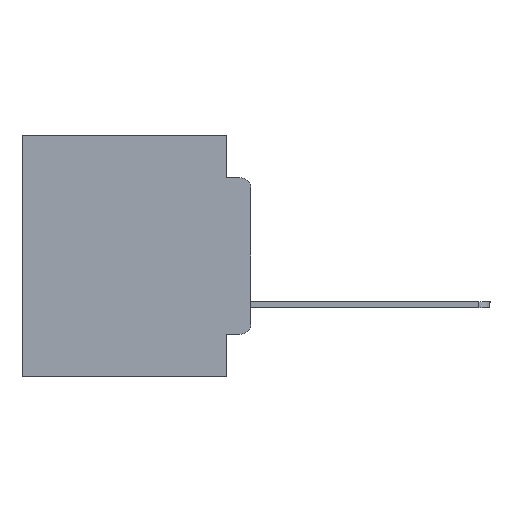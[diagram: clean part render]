
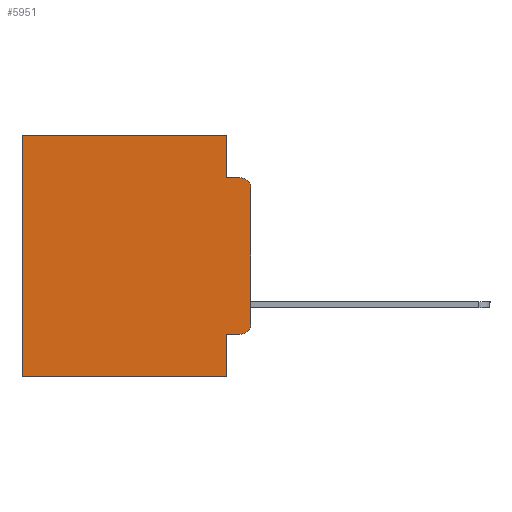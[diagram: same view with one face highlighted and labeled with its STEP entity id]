
A CAD part, left-side view. The second image highlights one B-rep face of the part: STEP entity #5951.
In plain terms, the highlighted planar face has unit normal (-1, 0, 0).
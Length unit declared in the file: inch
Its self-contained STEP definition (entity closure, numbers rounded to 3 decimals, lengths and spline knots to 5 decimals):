
#477 = CARTESIAN_POINT ( 'NONE',  ( 0.298, 0.051, -0.5 ) ) ;
#1164 = VECTOR ( 'NONE', #3734, 39.37008 ) ;
#1680 = ORIENTED_EDGE ( 'NONE', *, *, #22626, .F. ) ;
#1765 = VECTOR ( 'NONE', #3076, 39.37008 ) ;
#2395 = CARTESIAN_POINT ( 'NONE',  ( 0.298, 0.473, -0.5 ) ) ;
#2479 = DIRECTION ( 'NONE',  ( 0., 0., -1. ) ) ;
#2806 = VERTEX_POINT ( 'NONE', #5251 ) ;
#3076 = DIRECTION ( 'NONE',  ( 0., -1., 0. ) ) ;
#3149 = EDGE_CURVE ( 'NONE', #2806, #12710, #28818, .T. ) ;
#3280 = DIRECTION ( 'NONE',  ( -1., 0., 0. ) ) ;
#3322 = CARTESIAN_POINT ( 'NONE',  ( 0.298, 0.051, 0. ) ) ;
#3734 = DIRECTION ( 'NONE',  ( 0., 0., -1. ) ) ;
#3807 = PLANE ( 'NONE',  #22149 ) ;
#4066 = ORIENTED_EDGE ( 'NONE', *, *, #28423, .F. ) ;
#4563 = CARTESIAN_POINT ( 'NONE',  ( 0.298, 0., -0.3915 ) ) ;
#4841 = EDGE_CURVE ( 'NONE', #13880, #23480, #18587, .T. ) ;
#5045 = DIRECTION ( 'NONE',  ( -1., 0., 0. ) ) ;
#5251 = CARTESIAN_POINT ( 'NONE',  ( 0.298, 0., -0.1085 ) ) ;
#5495 = CARTESIAN_POINT ( 'NONE',  ( 0.298, 0., -0.5 ) ) ;
#5843 = DIRECTION ( 'NONE',  ( 0., 0., -1. ) ) ;
#5951 = ADVANCED_FACE ( 'NONE', ( #17304 ), #3807, .F. ) ;
#6473 = EDGE_CURVE ( 'NONE', #12694, #21999, #13450, .T. ) ;
#7042 = LINE ( 'NONE', #15993, #1765 ) ;
#9878 = AXIS2_PLACEMENT_3D ( 'NONE', #14836, #3280, #23289 ) ;
#10331 = CIRCLE ( 'NONE', #9878, 0.02 ) ;
#10466 = CARTESIAN_POINT ( 'NONE',  ( 0.298, 0.02, -0.0885 ) ) ;
#10479 = EDGE_CURVE ( 'NONE', #2806, #23607, #28975, .T. ) ;
#10748 = CARTESIAN_POINT ( 'NONE',  ( 0.298, 0., 0. ) ) ;
#11320 = EDGE_CURVE ( 'NONE', #13880, #13635, #14856, .T. ) ;
#12081 = ORIENTED_EDGE ( 'NONE', *, *, #4841, .T. ) ;
#12694 = VERTEX_POINT ( 'NONE', #14717 ) ;
#12710 = VERTEX_POINT ( 'NONE', #10466 ) ;
#12803 = LINE ( 'NONE', #10748, #27935 ) ;
#13104 = ORIENTED_EDGE ( 'NONE', *, *, #25873, .T. ) ;
#13133 = VECTOR ( 'NONE', #16226, 39.37008 ) ;
#13152 = CARTESIAN_POINT ( 'NONE',  ( 0.298, 0.473, 0. ) ) ;
#13450 = LINE ( 'NONE', #13152, #14121 ) ;
#13472 = CARTESIAN_POINT ( 'NONE',  ( 0.298, 0., 0. ) ) ;
#13635 = VERTEX_POINT ( 'NONE', #477 ) ;
#13880 = VERTEX_POINT ( 'NONE', #21483 ) ;
#14121 = VECTOR ( 'NONE', #22615, 39.37008 ) ;
#14569 = EDGE_CURVE ( 'NONE', #13635, #21999, #23181, .T. ) ;
#14702 = DIRECTION ( 'NONE',  ( 0., 1., 0. ) ) ;
#14717 = CARTESIAN_POINT ( 'NONE',  ( 0.298, 0.473, 0. ) ) ;
#14836 = CARTESIAN_POINT ( 'NONE',  ( 0.298, 0.02, -0.3915 ) ) ;
#14856 = LINE ( 'NONE', #17381, #1164 ) ;
#15084 = CARTESIAN_POINT ( 'NONE',  ( 0.298, 0., 0. ) ) ;
#15254 = CARTESIAN_POINT ( 'NONE',  ( 0.298, 0.02, -0.4115 ) ) ;
#15299 = ORIENTED_EDGE ( 'NONE', *, *, #14569, .F. ) ;
#15993 = CARTESIAN_POINT ( 'NONE',  ( 0.298, 0.051, -0.0885 ) ) ;
#16226 = DIRECTION ( 'NONE',  ( 0., -1., 0. ) ) ;
#16483 = DIRECTION ( 'NONE',  ( 0., 0., -1. ) ) ;
#17098 = ORIENTED_EDGE ( 'NONE', *, *, #6473, .T. ) ;
#17168 = CARTESIAN_POINT ( 'NONE',  ( 0.298, 0.051, -0.0885 ) ) ;
#17304 = FACE_OUTER_BOUND ( 'NONE', #22962, .T. ) ;
#17381 = CARTESIAN_POINT ( 'NONE',  ( 0.298, 0.051, 0. ) ) ;
#18193 = EDGE_CURVE ( 'NONE', #22625, #12694, #12803, .T. ) ;
#18293 = VECTOR ( 'NONE', #18473, 39.37008 ) ;
#18456 = AXIS2_PLACEMENT_3D ( 'NONE', #27041, #5045, #16483 ) ;
#18473 = DIRECTION ( 'NONE',  ( 0., 0., -1. ) ) ;
#18587 = LINE ( 'NONE', #25391, #13133 ) ;
#18737 = DIRECTION ( 'NONE',  ( 0., 1., 0. ) ) ;
#20976 = LINE ( 'NONE', #3322, #18293 ) ;
#21149 = CARTESIAN_POINT ( 'NONE',  ( 0.298, 0.051, 0. ) ) ;
#21483 = CARTESIAN_POINT ( 'NONE',  ( 0.298, 0.051, -0.4115 ) ) ;
#21999 = VERTEX_POINT ( 'NONE', #2395 ) ;
#22149 = AXIS2_PLACEMENT_3D ( 'NONE', #15084, #24113, #5843 ) ;
#22615 = DIRECTION ( 'NONE',  ( 0., 0., -1. ) ) ;
#22625 = VERTEX_POINT ( 'NONE', #21149 ) ;
#22626 = EDGE_CURVE ( 'NONE', #25217, #12710, #7042, .T. ) ;
#22962 = EDGE_LOOP ( 'NONE', ( #27747, #25265, #1680, #4066, #23292, #17098, #15299, #26859, #12081, #13104 ) ) ;
#23181 = LINE ( 'NONE', #5495, #26174 ) ;
#23289 = DIRECTION ( 'NONE',  ( 0., 0., -1. ) ) ;
#23292 = ORIENTED_EDGE ( 'NONE', *, *, #18193, .T. ) ;
#23480 = VERTEX_POINT ( 'NONE', #15254 ) ;
#23607 = VERTEX_POINT ( 'NONE', #4563 ) ;
#24113 = DIRECTION ( 'NONE',  ( 1., 0., 0. ) ) ;
#25217 = VERTEX_POINT ( 'NONE', #17168 ) ;
#25265 = ORIENTED_EDGE ( 'NONE', *, *, #3149, .T. ) ;
#25391 = CARTESIAN_POINT ( 'NONE',  ( 0.298, 0.051, -0.4115 ) ) ;
#25873 = EDGE_CURVE ( 'NONE', #23480, #23607, #10331, .T. ) ;
#26050 = VECTOR ( 'NONE', #2479, 39.37008 ) ;
#26174 = VECTOR ( 'NONE', #18737, 39.37008 ) ;
#26859 = ORIENTED_EDGE ( 'NONE', *, *, #11320, .F. ) ;
#27041 = CARTESIAN_POINT ( 'NONE',  ( 0.298, 0.02, -0.1085 ) ) ;
#27747 = ORIENTED_EDGE ( 'NONE', *, *, #10479, .F. ) ;
#27935 = VECTOR ( 'NONE', #14702, 39.37008 ) ;
#28423 = EDGE_CURVE ( 'NONE', #22625, #25217, #20976, .T. ) ;
#28818 = CIRCLE ( 'NONE', #18456, 0.02 ) ;
#28975 = LINE ( 'NONE', #13472, #26050 ) ;
